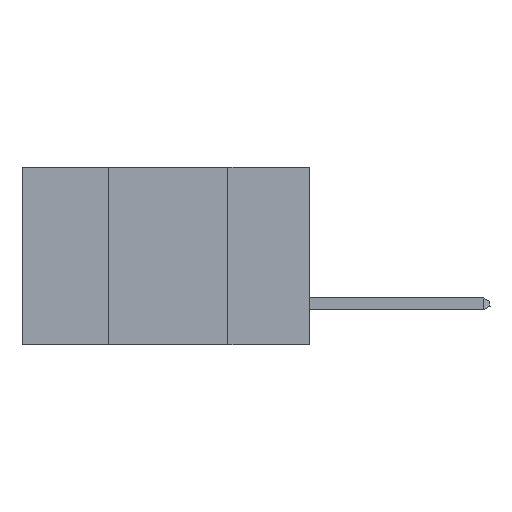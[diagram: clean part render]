
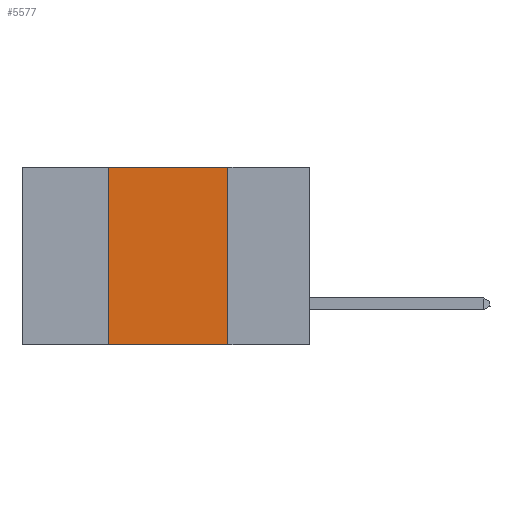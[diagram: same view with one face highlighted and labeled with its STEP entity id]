
A CAD part, left-side view. The second image highlights one B-rep face of the part: STEP entity #5577.
In plain terms, the highlighted planar face has unit normal (-1, 0, 0).
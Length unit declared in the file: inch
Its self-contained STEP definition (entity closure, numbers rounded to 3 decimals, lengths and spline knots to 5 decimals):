
#280 = ORIENTED_EDGE ( 'NONE', *, *, #8728, .F. ) ;
#407 = DIRECTION ( 'NONE',  ( 0., 0., -1. ) ) ;
#419 = LINE ( 'NONE', #11605, #11690 ) ;
#779 = CARTESIAN_POINT ( 'NONE',  ( 0., 0.17, -0.37 ) ) ;
#814 = EDGE_CURVE ( 'NONE', #2845, #967, #419, .T. ) ;
#846 = DIRECTION ( 'NONE',  ( 0., 0., -1. ) ) ;
#967 = VERTEX_POINT ( 'NONE', #7884 ) ;
#978 = EDGE_LOOP ( 'NONE', ( #2814, #280, #2460, #4776 ) ) ;
#1204 = VERTEX_POINT ( 'NONE', #6508 ) ;
#1253 = CARTESIAN_POINT ( 'NONE',  ( 0., 0.6, -0.37 ) ) ;
#1392 = CARTESIAN_POINT ( 'NONE',  ( 0., 0.6, 0. ) ) ;
#1920 = CARTESIAN_POINT ( 'NONE',  ( 0., 0.17, 0. ) ) ;
#2460 = ORIENTED_EDGE ( 'NONE', *, *, #814, .F. ) ;
#2814 = ORIENTED_EDGE ( 'NONE', *, *, #9931, .F. ) ;
#2845 = VERTEX_POINT ( 'NONE', #9215 ) ;
#3209 = FACE_OUTER_BOUND ( 'NONE', #978, .T. ) ;
#3319 = DIRECTION ( 'NONE',  ( 0., -1., 0. ) ) ;
#3409 = PLANE ( 'NONE',  #7290 ) ;
#4776 = ORIENTED_EDGE ( 'NONE', *, *, #11764, .T. ) ;
#5577 = ADVANCED_FACE ( 'NONE', ( #3209 ), #3409, .F. ) ;
#5694 = VECTOR ( 'NONE', #3319, 39.37008 ) ;
#6127 = LINE ( 'NONE', #1920, #10336 ) ;
#6181 = CARTESIAN_POINT ( 'NONE',  ( 0., 0.6, 0. ) ) ;
#6508 = CARTESIAN_POINT ( 'NONE',  ( 0., 0.17, 0. ) ) ;
#6856 = VECTOR ( 'NONE', #11342, 39.37008 ) ;
#7290 = AXIS2_PLACEMENT_3D ( 'NONE', #6181, #9066, #407 ) ;
#7884 = CARTESIAN_POINT ( 'NONE',  ( 0., 0.42, 0. ) ) ;
#8383 = VERTEX_POINT ( 'NONE', #779 ) ;
#8728 = EDGE_CURVE ( 'NONE', #967, #1204, #10503, .T. ) ;
#9066 = DIRECTION ( 'NONE',  ( 1., 0., 0. ) ) ;
#9215 = CARTESIAN_POINT ( 'NONE',  ( 0., 0.42, -0.37 ) ) ;
#9551 = LINE ( 'NONE', #1253, #6856 ) ;
#9931 = EDGE_CURVE ( 'NONE', #1204, #8383, #6127, .T. ) ;
#10336 = VECTOR ( 'NONE', #846, 39.37008 ) ;
#10503 = LINE ( 'NONE', #1392, #5694 ) ;
#10636 = DIRECTION ( 'NONE',  ( 0., 0., 1. ) ) ;
#11342 = DIRECTION ( 'NONE',  ( 0., -1., 0. ) ) ;
#11605 = CARTESIAN_POINT ( 'NONE',  ( 0., 0.42, 0. ) ) ;
#11690 = VECTOR ( 'NONE', #10636, 39.37008 ) ;
#11764 = EDGE_CURVE ( 'NONE', #2845, #8383, #9551, .T. ) ;
